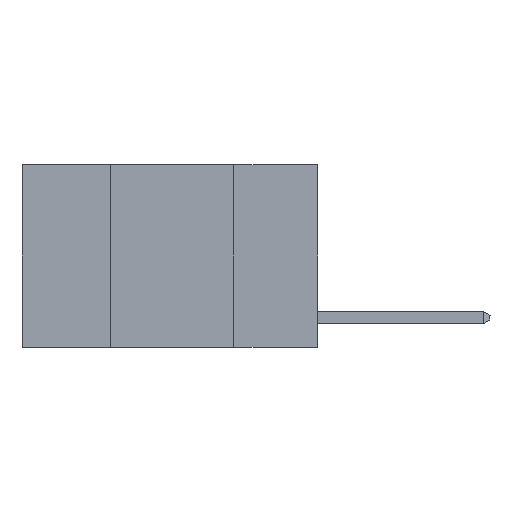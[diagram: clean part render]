
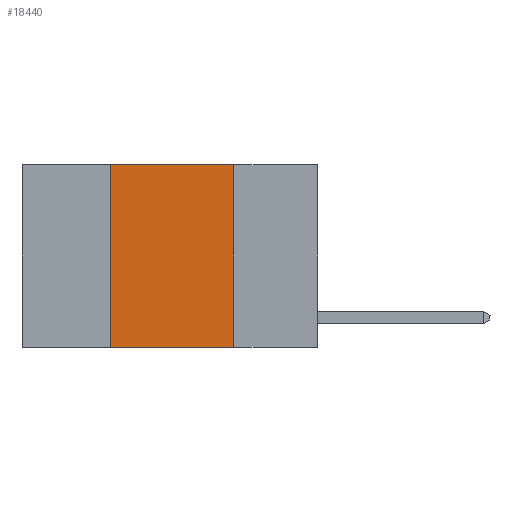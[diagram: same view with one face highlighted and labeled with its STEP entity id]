
A CAD part, left-side view. The second image highlights one B-rep face of the part: STEP entity #18440.
In plain terms, the highlighted planar face has unit normal (-1, 0, 0).
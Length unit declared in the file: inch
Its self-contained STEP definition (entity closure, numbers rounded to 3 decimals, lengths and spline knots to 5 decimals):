
#28 = LINE ( 'NONE', #15779, #15199 ) ;
#507 = VECTOR ( 'NONE', #7581, 39.37008 ) ;
#803 = CARTESIAN_POINT ( 'NONE',  ( 0., 0.6, -0.37 ) ) ;
#818 = ORIENTED_EDGE ( 'NONE', *, *, #2166, .F. ) ;
#2166 = EDGE_CURVE ( 'NONE', #12271, #4939, #7004, .T. ) ;
#3134 = ORIENTED_EDGE ( 'NONE', *, *, #3713, .F. ) ;
#3713 = EDGE_CURVE ( 'NONE', #4939, #7488, #28, .T. ) ;
#3902 = DIRECTION ( 'NONE',  ( 0., 0., -1. ) ) ;
#4570 = ORIENTED_EDGE ( 'NONE', *, *, #8402, .F. ) ;
#4939 = VERTEX_POINT ( 'NONE', #5161 ) ;
#5161 = CARTESIAN_POINT ( 'NONE',  ( 0., 0.42, 0. ) ) ;
#5891 = CARTESIAN_POINT ( 'NONE',  ( 0., 0.42, -0.37 ) ) ;
#6337 = VECTOR ( 'NONE', #16026, 39.37008 ) ;
#6447 = VECTOR ( 'NONE', #16575, 39.37008 ) ;
#7004 = LINE ( 'NONE', #13315, #6337 ) ;
#7488 = VERTEX_POINT ( 'NONE', #11176 ) ;
#7581 = DIRECTION ( 'NONE',  ( 0., 0., -1. ) ) ;
#8178 = DIRECTION ( 'NONE',  ( 1., 0., 0. ) ) ;
#8179 = CARTESIAN_POINT ( 'NONE',  ( 0., 0.17, -0.37 ) ) ;
#8402 = EDGE_CURVE ( 'NONE', #7488, #13666, #11891, .T. ) ;
#8816 = DIRECTION ( 'NONE',  ( 0., -1., 0. ) ) ;
#8869 = ORIENTED_EDGE ( 'NONE', *, *, #10584, .T. ) ;
#10584 = EDGE_CURVE ( 'NONE', #12271, #13666, #13123, .T. ) ;
#11163 = EDGE_LOOP ( 'NONE', ( #4570, #3134, #818, #8869 ) ) ;
#11176 = CARTESIAN_POINT ( 'NONE',  ( 0., 0.17, 0. ) ) ;
#11710 = AXIS2_PLACEMENT_3D ( 'NONE', #12305, #8178, #3902 ) ;
#11891 = LINE ( 'NONE', #13204, #507 ) ;
#12271 = VERTEX_POINT ( 'NONE', #5891 ) ;
#12305 = CARTESIAN_POINT ( 'NONE',  ( 0., 0.6, 0. ) ) ;
#13123 = LINE ( 'NONE', #803, #6447 ) ;
#13204 = CARTESIAN_POINT ( 'NONE',  ( 0., 0.17, 0. ) ) ;
#13315 = CARTESIAN_POINT ( 'NONE',  ( 0., 0.42, 0. ) ) ;
#13666 = VERTEX_POINT ( 'NONE', #8179 ) ;
#15199 = VECTOR ( 'NONE', #8816, 39.37008 ) ;
#15370 = PLANE ( 'NONE',  #11710 ) ;
#15779 = CARTESIAN_POINT ( 'NONE',  ( 0., 0.6, 0. ) ) ;
#15863 = FACE_OUTER_BOUND ( 'NONE', #11163, .T. ) ;
#16026 = DIRECTION ( 'NONE',  ( 0., 0., 1. ) ) ;
#16575 = DIRECTION ( 'NONE',  ( 0., -1., 0. ) ) ;
#18440 = ADVANCED_FACE ( 'NONE', ( #15863 ), #15370, .F. ) ;
